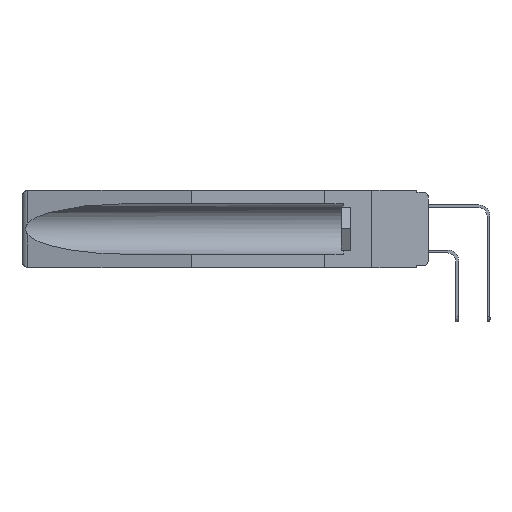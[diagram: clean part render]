
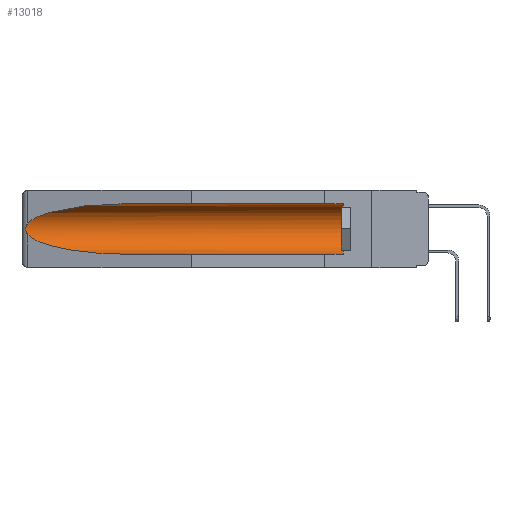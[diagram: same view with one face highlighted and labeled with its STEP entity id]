
A CAD part, left-side view. The second image highlights one B-rep face of the part: STEP entity #13018.
In plain terms, the highlighted cylindrical face has radius 2.857 mm (diameter 5.715 mm), a partial arc.
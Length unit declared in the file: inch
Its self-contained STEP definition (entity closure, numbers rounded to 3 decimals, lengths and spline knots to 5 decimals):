
#483 = CARTESIAN_POINT ( 'NONE',  ( 0.2675, 1.53308, -0.16763 ) ) ;
#639 = CARTESIAN_POINT ( 'NONE',  ( 0.26537, 1.52718, -0.19328 ) ) ;
#2193 = EDGE_CURVE ( 'NONE', #6559, #17653, #11392, .T. ) ;
#2386 = CARTESIAN_POINT ( 'NONE',  ( 0.25451, 1.48313, -0.24835 ) ) ;
#2627 = CARTESIAN_POINT ( 'NONE',  ( 0.26654, 1.53092, -0.15636 ) ) ;
#3067 = CARTESIAN_POINT ( 'NONE',  ( 0.155, 1.07973, -0.284 ) ) ;
#3245 = AXIS2_PLACEMENT_3D ( 'NONE', #7943, #16659, #5801 ) ;
#3321 = CARTESIAN_POINT ( 'NONE',  ( 0.21114, 1.30732, -0.059 ) ) ;
#3482 = ORIENTED_EDGE ( 'NONE', *, *, #3874, .T. ) ;
#3612 = CARTESIAN_POINT ( 'NONE',  ( 0.155, 0.126, -0.284 ) ) ;
#3874 = EDGE_CURVE ( 'NONE', #7255, #23687, #9118, .T. ) ;
#3900 = EDGE_CURVE ( 'NONE', #22467, #23687, #18100, .T. ) ;
#4914 = CARTESIAN_POINT ( 'NONE',  ( 0.26537, 1.52718, -0.14972 ) ) ;
#4975 = DIRECTION ( 'NONE',  ( 0., 1., 0. ) ) ;
#5034 = VERTEX_POINT ( 'NONE', #18817 ) ;
#5401 = ORIENTED_EDGE ( 'NONE', *, *, #12056, .T. ) ;
#5801 = DIRECTION ( 'NONE',  ( 0., 0., 1. ) ) ;
#6559 = VERTEX_POINT ( 'NONE', #17514 ) ;
#7126 = VECTOR ( 'NONE', #4975, 39.37008 ) ;
#7255 = VERTEX_POINT ( 'NONE', #18330 ) ;
#7608 = EDGE_LOOP ( 'NONE', ( #22920, #5401, #3482, #14900, #23896, #11971 ) ) ;
#7696 = CARTESIAN_POINT ( 'NONE',  ( 0.155, 1.07973, -0.059 ) ) ;
#7943 = CARTESIAN_POINT ( 'NONE',  ( 0.155, -0.30754, -0.1715 ) ) ;
#8310 = EDGE_CURVE ( 'NONE', #22467, #6559, #22882, .T. ) ;
#9098 = VECTOR ( 'NONE', #9247, 39.37008 ) ;
#9118 =( BOUNDED_CURVE ( )  B_SPLINE_CURVE ( 3, ( #21966, #2386, #18233, #13523 ),
 .UNSPECIFIED., .F., .T. ) 
 B_SPLINE_CURVE_WITH_KNOTS ( ( 4, 4 ),
 ( 0.1948, 1.5708 ),
 .UNSPECIFIED. ) 
 CURVE ( )  GEOMETRIC_REPRESENTATION_ITEM ( )  RATIONAL_B_SPLINE_CURVE ( ( 1., 0.848, 0.848, 1. ) ) 
 REPRESENTATION_ITEM ( '' )  );
#9247 = DIRECTION ( 'NONE',  ( 0., 1., 0. ) ) ;
#9451 = CARTESIAN_POINT ( 'NONE',  ( 0.155, 1.07973, -0.059 ) ) ;
#9578 = B_SPLINE_CURVE_WITH_KNOTS ( 'NONE', 3,
 ( #4914, #22219, #2627, #20062, #483, #22350, #17923, #19792, #15782, #639 ),
 .UNSPECIFIED., .F., .F.,
 ( 4, 2, 2, 2, 4 ),
 ( 0., 0.00029, 0.00058, 0.00087, 0.00117 ),
 .UNSPECIFIED. ) ;
#9872 = CARTESIAN_POINT ( 'NONE',  ( 0.26537, 1.52718, -0.14972 ) ) ;
#10102 = CARTESIAN_POINT ( 'NONE',  ( 0.155, 0.126, -0.1715 ) ) ;
#10208 =( BOUNDED_CURVE ( )  B_SPLINE_CURVE ( 3, ( #9451, #3321, #18457, #9872 ),
 .UNSPECIFIED., .F., .T. ) 
 B_SPLINE_CURVE_WITH_KNOTS ( ( 4, 4 ),
 ( 4.71239, 6.08839 ),
 .UNSPECIFIED. ) 
 CURVE ( )  GEOMETRIC_REPRESENTATION_ITEM ( )  RATIONAL_B_SPLINE_CURVE ( ( 1., 0.848, 0.848, 1. ) ) 
 REPRESENTATION_ITEM ( '' )  );
#10226 = FACE_OUTER_BOUND ( 'NONE', #7608, .T. ) ;
#11392 = LINE ( 'NONE', #11552, #7126 ) ;
#11458 = AXIS2_PLACEMENT_3D ( 'NONE', #10102, #20828, #14818 ) ;
#11526 = CARTESIAN_POINT ( 'NONE',  ( 0.155, -0.30754, -0.284 ) ) ;
#11552 = CARTESIAN_POINT ( 'NONE',  ( 0.155, -0.30754, -0.059 ) ) ;
#11942 = CYLINDRICAL_SURFACE ( 'NONE', #3245, 0.1125 ) ;
#11971 = ORIENTED_EDGE ( 'NONE', *, *, #2193, .T. ) ;
#12056 = EDGE_CURVE ( 'NONE', #5034, #7255, #9578, .T. ) ;
#13018 = ADVANCED_FACE ( 'NONE', ( #10226 ), #11942, .F. ) ;
#13523 = CARTESIAN_POINT ( 'NONE',  ( 0.155, 1.07973, -0.284 ) ) ;
#14818 = DIRECTION ( 'NONE',  ( 0., 0., 1. ) ) ;
#14900 = ORIENTED_EDGE ( 'NONE', *, *, #3900, .F. ) ;
#15782 = CARTESIAN_POINT ( 'NONE',  ( 0.26597, 1.5296, -0.19026 ) ) ;
#16659 = DIRECTION ( 'NONE',  ( 0., 1., 0. ) ) ;
#17514 = CARTESIAN_POINT ( 'NONE',  ( 0.155, 0.126, -0.059 ) ) ;
#17653 = VERTEX_POINT ( 'NONE', #7696 ) ;
#17923 = CARTESIAN_POINT ( 'NONE',  ( 0.2673, 1.53269, -0.17917 ) ) ;
#18100 = LINE ( 'NONE', #11526, #9098 ) ;
#18233 = CARTESIAN_POINT ( 'NONE',  ( 0.21114, 1.30732, -0.284 ) ) ;
#18330 = CARTESIAN_POINT ( 'NONE',  ( 0.26537, 1.52718, -0.19328 ) ) ;
#18457 = CARTESIAN_POINT ( 'NONE',  ( 0.25451, 1.48313, -0.09465 ) ) ;
#18817 = CARTESIAN_POINT ( 'NONE',  ( 0.26537, 1.52718, -0.14972 ) ) ;
#19792 = CARTESIAN_POINT ( 'NONE',  ( 0.26655, 1.53094, -0.18657 ) ) ;
#20062 = CARTESIAN_POINT ( 'NONE',  ( 0.2673, 1.5327, -0.16383 ) ) ;
#20828 = DIRECTION ( 'NONE',  ( 0., -1., 0. ) ) ;
#21966 = CARTESIAN_POINT ( 'NONE',  ( 0.26537, 1.52718, -0.19328 ) ) ;
#22219 = CARTESIAN_POINT ( 'NONE',  ( 0.26597, 1.52961, -0.15275 ) ) ;
#22350 = CARTESIAN_POINT ( 'NONE',  ( 0.2675, 1.53308, -0.17534 ) ) ;
#22467 = VERTEX_POINT ( 'NONE', #3612 ) ;
#22882 = CIRCLE ( 'NONE', #11458, 0.1125 ) ;
#22920 = ORIENTED_EDGE ( 'NONE', *, *, #24247, .T. ) ;
#23687 = VERTEX_POINT ( 'NONE', #3067 ) ;
#23896 = ORIENTED_EDGE ( 'NONE', *, *, #8310, .T. ) ;
#24247 = EDGE_CURVE ( 'NONE', #17653, #5034, #10208, .T. ) ;
